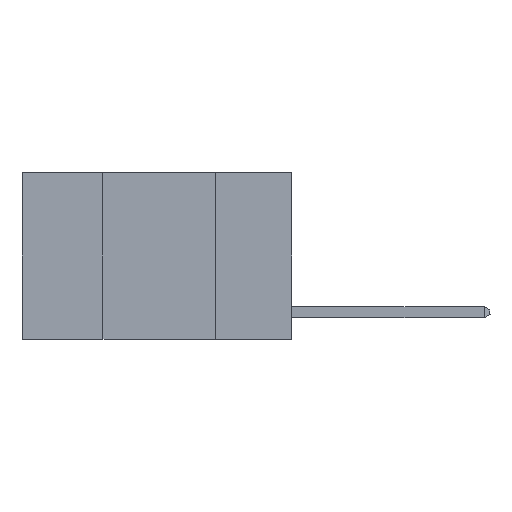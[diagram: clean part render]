
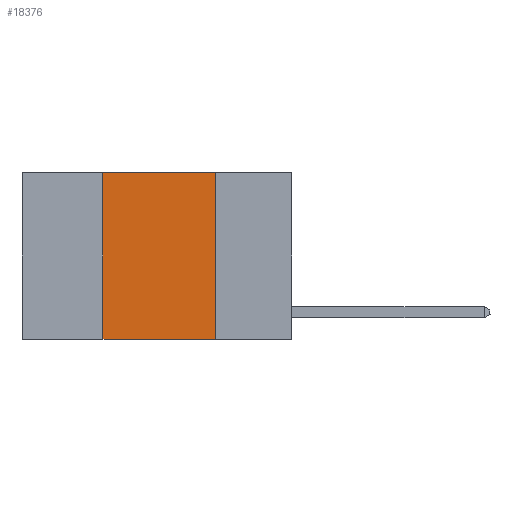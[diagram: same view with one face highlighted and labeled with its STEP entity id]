
A CAD part, left-side view. The second image highlights one B-rep face of the part: STEP entity #18376.
In plain terms, the highlighted planar face has unit normal (-1, 0, 0).
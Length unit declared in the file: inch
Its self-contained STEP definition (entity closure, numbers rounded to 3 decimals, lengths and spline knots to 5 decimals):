
#996 = CARTESIAN_POINT ( 'NONE',  ( 0., 0.17, 0. ) ) ;
#1192 = DIRECTION ( 'NONE',  ( 1., 0., 0. ) ) ;
#1245 = VERTEX_POINT ( 'NONE', #7241 ) ;
#1987 = LINE ( 'NONE', #15124, #16484 ) ;
#2097 = EDGE_CURVE ( 'NONE', #15378, #1245, #18730, .T. ) ;
#2827 = CARTESIAN_POINT ( 'NONE',  ( 0., 0.42, -0.37 ) ) ;
#3277 = CARTESIAN_POINT ( 'NONE',  ( 0., 0.6, 0. ) ) ;
#3529 = CARTESIAN_POINT ( 'NONE',  ( 0., 0.17, -0.37 ) ) ;
#3606 = LINE ( 'NONE', #3277, #19605 ) ;
#4047 = ORIENTED_EDGE ( 'NONE', *, *, #12753, .T. ) ;
#4231 = CARTESIAN_POINT ( 'NONE',  ( 0., 0.6, 0. ) ) ;
#4483 = VERTEX_POINT ( 'NONE', #3529 ) ;
#5402 = AXIS2_PLACEMENT_3D ( 'NONE', #4231, #1192, #17661 ) ;
#5941 = DIRECTION ( 'NONE',  ( 0., 0., 1. ) ) ;
#7064 = ORIENTED_EDGE ( 'NONE', *, *, #16663, .F. ) ;
#7241 = CARTESIAN_POINT ( 'NONE',  ( 0., 0.42, 0. ) ) ;
#7759 = EDGE_CURVE ( 'NONE', #1245, #16732, #3606, .T. ) ;
#8435 = DIRECTION ( 'NONE',  ( 0., -1., 0. ) ) ;
#8939 = EDGE_LOOP ( 'NONE', ( #7064, #9861, #10012, #4047 ) ) ;
#9382 = FACE_OUTER_BOUND ( 'NONE', #8939, .T. ) ;
#9861 = ORIENTED_EDGE ( 'NONE', *, *, #7759, .F. ) ;
#10011 = VECTOR ( 'NONE', #12528, 39.37008 ) ;
#10012 = ORIENTED_EDGE ( 'NONE', *, *, #2097, .F. ) ;
#10904 = CARTESIAN_POINT ( 'NONE',  ( 0., 0.17, 0. ) ) ;
#11674 = DIRECTION ( 'NONE',  ( 0., -1., 0. ) ) ;
#12528 = DIRECTION ( 'NONE',  ( 0., 0., -1. ) ) ;
#12609 = CARTESIAN_POINT ( 'NONE',  ( 0., 0.42, 0. ) ) ;
#12753 = EDGE_CURVE ( 'NONE', #15378, #4483, #1987, .T. ) ;
#15124 = CARTESIAN_POINT ( 'NONE',  ( 0., 0.6, -0.37 ) ) ;
#15378 = VERTEX_POINT ( 'NONE', #2827 ) ;
#15957 = PLANE ( 'NONE',  #5402 ) ;
#16484 = VECTOR ( 'NONE', #8435, 39.37008 ) ;
#16663 = EDGE_CURVE ( 'NONE', #16732, #4483, #20698, .T. ) ;
#16732 = VERTEX_POINT ( 'NONE', #996 ) ;
#17443 = VECTOR ( 'NONE', #5941, 39.37008 ) ;
#17661 = DIRECTION ( 'NONE',  ( 0., 0., -1. ) ) ;
#18376 = ADVANCED_FACE ( 'NONE', ( #9382 ), #15957, .F. ) ;
#18730 = LINE ( 'NONE', #12609, #17443 ) ;
#19605 = VECTOR ( 'NONE', #11674, 39.37008 ) ;
#20698 = LINE ( 'NONE', #10904, #10011 ) ;
